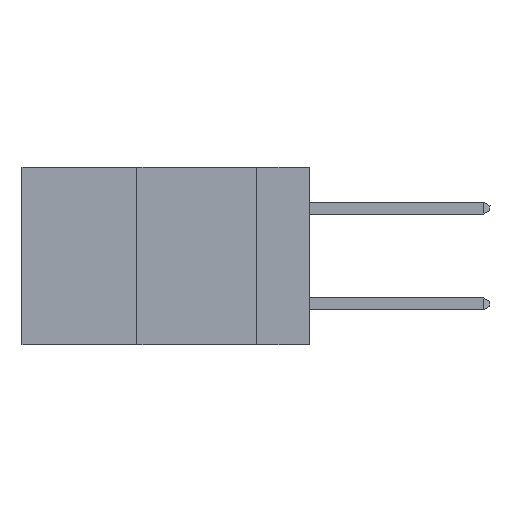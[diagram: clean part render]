
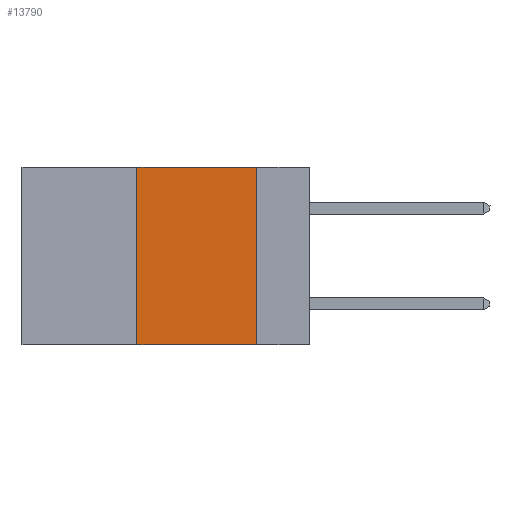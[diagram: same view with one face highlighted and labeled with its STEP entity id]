
A CAD part, left-side view. The second image highlights one B-rep face of the part: STEP entity #13790.
In plain terms, the highlighted planar face has unit normal (-1, 0, 0).
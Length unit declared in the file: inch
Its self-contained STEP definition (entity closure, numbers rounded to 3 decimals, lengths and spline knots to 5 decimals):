
#589 = DIRECTION ( 'NONE',  ( 0., 0., 1. ) ) ;
#1348 = CARTESIAN_POINT ( 'NONE',  ( 0., 0.36, 0. ) ) ;
#1352 = EDGE_CURVE ( 'NONE', #7845, #10005, #1910, .T. ) ;
#1504 = VERTEX_POINT ( 'NONE', #14814 ) ;
#1558 = ORIENTED_EDGE ( 'NONE', *, *, #9432, .F. ) ;
#1602 = FACE_OUTER_BOUND ( 'NONE', #5482, .T. ) ;
#1781 = CARTESIAN_POINT ( 'NONE',  ( 0., 0.6, 0. ) ) ;
#1910 = LINE ( 'NONE', #8103, #4944 ) ;
#2023 = VECTOR ( 'NONE', #3927, 39.37008 ) ;
#2267 = VERTEX_POINT ( 'NONE', #3082 ) ;
#2403 = LINE ( 'NONE', #11498, #2023 ) ;
#2521 = CARTESIAN_POINT ( 'NONE',  ( 0., 0.36, -0.37 ) ) ;
#3005 = EDGE_CURVE ( 'NONE', #7845, #2267, #11209, .T. ) ;
#3082 = CARTESIAN_POINT ( 'NONE',  ( 0., 0.36, 0. ) ) ;
#3190 = DIRECTION ( 'NONE',  ( 0., -1., 0. ) ) ;
#3310 = ORIENTED_EDGE ( 'NONE', *, *, #3005, .F. ) ;
#3927 = DIRECTION ( 'NONE',  ( 0., -1., 0. ) ) ;
#4215 = PLANE ( 'NONE',  #8841 ) ;
#4944 = VECTOR ( 'NONE', #3190, 39.37008 ) ;
#5263 = DIRECTION ( 'NONE',  ( 0., 0., -1. ) ) ;
#5370 = DIRECTION ( 'NONE',  ( 0., 0., -1. ) ) ;
#5482 = EDGE_LOOP ( 'NONE', ( #1558, #8195, #3310, #6354 ) ) ;
#6023 = EDGE_CURVE ( 'NONE', #2267, #1504, #2403, .T. ) ;
#6354 = ORIENTED_EDGE ( 'NONE', *, *, #1352, .T. ) ;
#7300 = LINE ( 'NONE', #11006, #10708 ) ;
#7845 = VERTEX_POINT ( 'NONE', #2521 ) ;
#8103 = CARTESIAN_POINT ( 'NONE',  ( 0., 0.6, -0.37 ) ) ;
#8195 = ORIENTED_EDGE ( 'NONE', *, *, #6023, .F. ) ;
#8557 = CARTESIAN_POINT ( 'NONE',  ( 0., 0.11, -0.37 ) ) ;
#8841 = AXIS2_PLACEMENT_3D ( 'NONE', #1781, #12246, #5370 ) ;
#9432 = EDGE_CURVE ( 'NONE', #1504, #10005, #7300, .T. ) ;
#10005 = VERTEX_POINT ( 'NONE', #8557 ) ;
#10708 = VECTOR ( 'NONE', #5263, 39.37008 ) ;
#11006 = CARTESIAN_POINT ( 'NONE',  ( 0., 0.11, 0. ) ) ;
#11209 = LINE ( 'NONE', #1348, #14136 ) ;
#11498 = CARTESIAN_POINT ( 'NONE',  ( 0., 0.6, 0. ) ) ;
#12246 = DIRECTION ( 'NONE',  ( 1., 0., 0. ) ) ;
#13790 = ADVANCED_FACE ( 'NONE', ( #1602 ), #4215, .F. ) ;
#14136 = VECTOR ( 'NONE', #589, 39.37008 ) ;
#14814 = CARTESIAN_POINT ( 'NONE',  ( 0., 0.11, 0. ) ) ;
